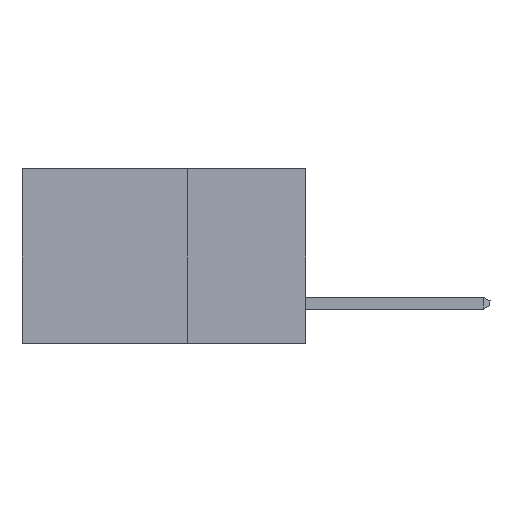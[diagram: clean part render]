
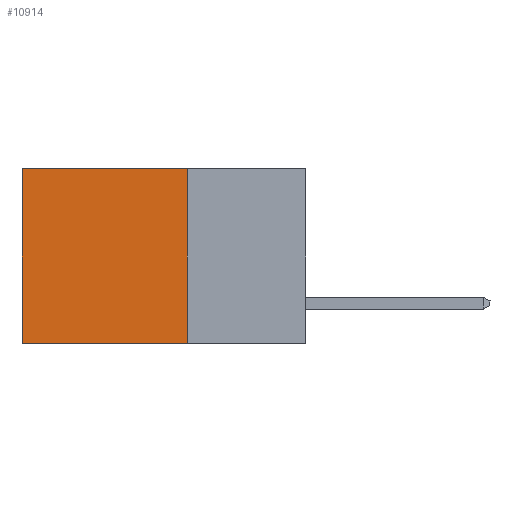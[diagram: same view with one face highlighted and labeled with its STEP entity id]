
A CAD part, left-side view. The second image highlights one B-rep face of the part: STEP entity #10914.
In plain terms, the highlighted planar face has unit normal (-1, 0, 0).
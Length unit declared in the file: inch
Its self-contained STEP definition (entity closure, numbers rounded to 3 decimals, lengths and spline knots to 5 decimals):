
#316 = VECTOR ( 'NONE', #7946, 39.37008 ) ;
#322 = CARTESIAN_POINT ( 'NONE',  ( 0.2615, 0.25, -0.37 ) ) ;
#842 = CARTESIAN_POINT ( 'NONE',  ( 0.2615, 0.25, -0.37 ) ) ;
#1070 = VECTOR ( 'NONE', #11254, 39.37008 ) ;
#1161 = EDGE_CURVE ( 'NONE', #12000, #11147, #3880, .T. ) ;
#1314 = LINE ( 'NONE', #322, #1070 ) ;
#2662 = ORIENTED_EDGE ( 'NONE', *, *, #3598, .T. ) ;
#3031 = DIRECTION ( 'NONE',  ( 0., 0., -1. ) ) ;
#3598 = EDGE_CURVE ( 'NONE', #11147, #5045, #9088, .T. ) ;
#3880 = LINE ( 'NONE', #11211, #316 ) ;
#5045 = VERTEX_POINT ( 'NONE', #10177 ) ;
#5083 = EDGE_LOOP ( 'NONE', ( #2662, #6282, #12574, #8725 ) ) ;
#6094 = CARTESIAN_POINT ( 'NONE',  ( 0.2615, 0.6, 0. ) ) ;
#6244 = DIRECTION ( 'NONE',  ( 1., 0., 0. ) ) ;
#6282 = ORIENTED_EDGE ( 'NONE', *, *, #9289, .F. ) ;
#6994 = CARTESIAN_POINT ( 'NONE',  ( 0.2615, 0.25, -0.37 ) ) ;
#7183 = CARTESIAN_POINT ( 'NONE',  ( 0.2615, 0.25, 0. ) ) ;
#7306 = FACE_OUTER_BOUND ( 'NONE', #5083, .T. ) ;
#7771 = VERTEX_POINT ( 'NONE', #6994 ) ;
#7842 = DIRECTION ( 'NONE',  ( 0., 0., -1. ) ) ;
#7897 = LINE ( 'NONE', #842, #11266 ) ;
#7946 = DIRECTION ( 'NONE',  ( 0., 1., 0. ) ) ;
#8108 = AXIS2_PLACEMENT_3D ( 'NONE', #10433, #6244, #9298 ) ;
#8425 = VECTOR ( 'NONE', #7842, 39.37008 ) ;
#8614 = EDGE_CURVE ( 'NONE', #12000, #7771, #7897, .T. ) ;
#8725 = ORIENTED_EDGE ( 'NONE', *, *, #1161, .T. ) ;
#9088 = LINE ( 'NONE', #11972, #8425 ) ;
#9289 = EDGE_CURVE ( 'NONE', #7771, #5045, #1314, .T. ) ;
#9298 = DIRECTION ( 'NONE',  ( 0., 0., -1. ) ) ;
#10177 = CARTESIAN_POINT ( 'NONE',  ( 0.2615, 0.6, -0.37 ) ) ;
#10246 = PLANE ( 'NONE',  #8108 ) ;
#10433 = CARTESIAN_POINT ( 'NONE',  ( 0.2615, 0.25, -0.37 ) ) ;
#10914 = ADVANCED_FACE ( 'NONE', ( #7306 ), #10246, .F. ) ;
#11147 = VERTEX_POINT ( 'NONE', #6094 ) ;
#11211 = CARTESIAN_POINT ( 'NONE',  ( 0.2615, 0.25, 0. ) ) ;
#11254 = DIRECTION ( 'NONE',  ( 0., 1., 0. ) ) ;
#11266 = VECTOR ( 'NONE', #3031, 39.37008 ) ;
#11972 = CARTESIAN_POINT ( 'NONE',  ( 0.2615, 0.6, -0.37 ) ) ;
#12000 = VERTEX_POINT ( 'NONE', #7183 ) ;
#12574 = ORIENTED_EDGE ( 'NONE', *, *, #8614, .F. ) ;
